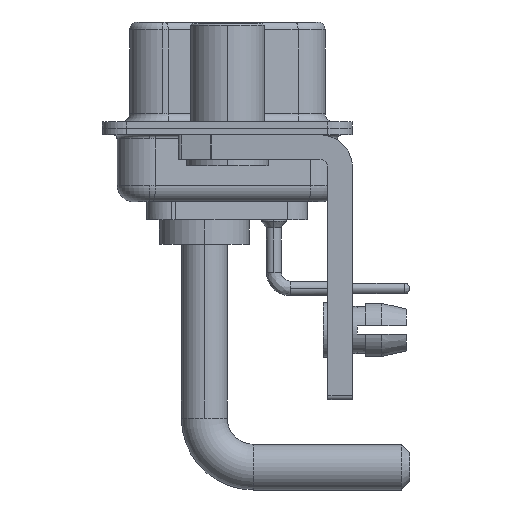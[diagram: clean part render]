
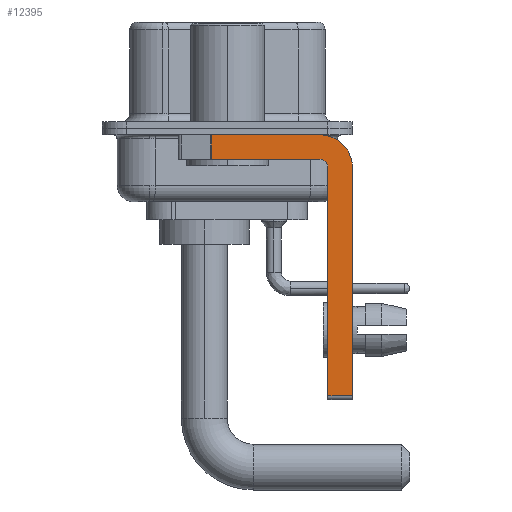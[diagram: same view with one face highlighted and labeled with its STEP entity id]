
A CAD part, left-side view. The second image highlights one B-rep face of the part: STEP entity #12395.
In plain terms, the highlighted planar face has unit normal (-1, 0, 0).
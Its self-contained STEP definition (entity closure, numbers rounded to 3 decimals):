
#335 = VECTOR ( 'NONE', #17291, 1000. ) ;
#448 = VECTOR ( 'NONE', #26796, 1000. ) ;
#1415 = AXIS2_PLACEMENT_3D ( 'NONE', #9106, #7121, #15744 ) ;
#1646 = LINE ( 'NONE', #10288, #11761 ) ;
#1775 = CARTESIAN_POINT ( 'NONE',  ( -2.9, -7.65, -2.4 ) ) ;
#2487 = ORIENTED_EDGE ( 'NONE', *, *, #11642, .F. ) ;
#3625 = AXIS2_PLACEMENT_3D ( 'NONE', #11857, #13549, #9172 ) ;
#4670 = LINE ( 'NONE', #25917, #10316 ) ;
#4690 = VERTEX_POINT ( 'NONE', #8998 ) ;
#4702 = EDGE_CURVE ( 'NONE', #9574, #25450, #22022, .T. ) ;
#4993 = CIRCLE ( 'NONE', #1415, 2. ) ;
#5126 = VERTEX_POINT ( 'NONE', #18393 ) ;
#7117 = EDGE_LOOP ( 'NONE', ( #9124, #17147, #12365, #19292, #2487, #23918, #9658, #9670 ) ) ;
#7121 = DIRECTION ( 'NONE',  ( 1., 0., 0. ) ) ;
#7464 = PLANE ( 'NONE',  #3625 ) ;
#8009 = DIRECTION ( 'NONE',  ( -1., 0., 0. ) ) ;
#8576 = DIRECTION ( 'NONE',  ( 0., -1., 0. ) ) ;
#8673 = CARTESIAN_POINT ( 'NONE',  ( -2.9, -5.65, -16.35 ) ) ;
#8998 = CARTESIAN_POINT ( 'NONE',  ( -2.9, 0.978, -1.9 ) ) ;
#9106 = CARTESIAN_POINT ( 'NONE',  ( -2.9, -5.65, -2.4 ) ) ;
#9124 = ORIENTED_EDGE ( 'NONE', *, *, #13125, .F. ) ;
#9172 = DIRECTION ( 'NONE',  ( 0., 0., -1. ) ) ;
#9574 = VERTEX_POINT ( 'NONE', #1775 ) ;
#9658 = ORIENTED_EDGE ( 'NONE', *, *, #4702, .F. ) ;
#9670 = ORIENTED_EDGE ( 'NONE', *, *, #26041, .F. ) ;
#10172 = VERTEX_POINT ( 'NONE', #19708 ) ;
#10288 = CARTESIAN_POINT ( 'NONE',  ( -2.9, 3., -0.4 ) ) ;
#10316 = VECTOR ( 'NONE', #13300, 1000. ) ;
#11395 = VERTEX_POINT ( 'NONE', #25543 ) ;
#11642 = EDGE_CURVE ( 'NONE', #5126, #10172, #13886, .T. ) ;
#11761 = VECTOR ( 'NONE', #8576, 1000. ) ;
#11857 = CARTESIAN_POINT ( 'NONE',  ( -2.9, -5.65, -2.4 ) ) ;
#11961 = DIRECTION ( 'NONE',  ( 0., 0., -1. ) ) ;
#12365 = ORIENTED_EDGE ( 'NONE', *, *, #17684, .F. ) ;
#12395 = ADVANCED_FACE ( 'NONE', ( #20202 ), #7464, .F. ) ;
#13125 = EDGE_CURVE ( 'NONE', #26053, #11395, #1646, .T. ) ;
#13178 = VECTOR ( 'NONE', #11961, 1000. ) ;
#13300 = DIRECTION ( 'NONE',  ( 0., 1., 0. ) ) ;
#13549 = DIRECTION ( 'NONE',  ( 1., 0., 0. ) ) ;
#13759 = CARTESIAN_POINT ( 'NONE',  ( -2.9, -6.15, -16.6 ) ) ;
#13886 = LINE ( 'NONE', #13759, #448 ) ;
#15744 = DIRECTION ( 'NONE',  ( 0., 0., -1. ) ) ;
#15843 = EDGE_CURVE ( 'NONE', #26053, #4690, #19353, .T. ) ;
#15903 = VECTOR ( 'NONE', #26146, 1000. ) ;
#17147 = ORIENTED_EDGE ( 'NONE', *, *, #15843, .T. ) ;
#17173 = EDGE_CURVE ( 'NONE', #5126, #25450, #26367, .T. ) ;
#17198 = CARTESIAN_POINT ( 'NONE',  ( -2.9, -7.65, -16.35 ) ) ;
#17291 = DIRECTION ( 'NONE',  ( 0., -1., 0. ) ) ;
#17684 = EDGE_CURVE ( 'NONE', #19979, #4690, #4670, .T. ) ;
#18155 = CARTESIAN_POINT ( 'NONE',  ( -2.9, 0.978, -0.4 ) ) ;
#18393 = CARTESIAN_POINT ( 'NONE',  ( -2.9, -6.15, -16.35 ) ) ;
#18909 = CARTESIAN_POINT ( 'NONE',  ( -2.9, -5.65, -2.4 ) ) ;
#19292 = ORIENTED_EDGE ( 'NONE', *, *, #23927, .F. ) ;
#19353 = LINE ( 'NONE', #24034, #15903 ) ;
#19708 = CARTESIAN_POINT ( 'NONE',  ( -2.9, -6.15, -2.4 ) ) ;
#19979 = VERTEX_POINT ( 'NONE', #25011 ) ;
#20202 = FACE_OUTER_BOUND ( 'NONE', #7117, .T. ) ;
#22022 = LINE ( 'NONE', #25128, #13178 ) ;
#22883 = DIRECTION ( 'NONE',  ( 0., 0., 1. ) ) ;
#23918 = ORIENTED_EDGE ( 'NONE', *, *, #17173, .T. ) ;
#23927 = EDGE_CURVE ( 'NONE', #10172, #19979, #24711, .T. ) ;
#24034 = CARTESIAN_POINT ( 'NONE',  ( -2.9, 0.978, -1.9 ) ) ;
#24711 = CIRCLE ( 'NONE', #27431, 0.5 ) ;
#25011 = CARTESIAN_POINT ( 'NONE',  ( -2.9, -5.65, -1.9 ) ) ;
#25128 = CARTESIAN_POINT ( 'NONE',  ( -2.9, -7.65, -2.4 ) ) ;
#25450 = VERTEX_POINT ( 'NONE', #17198 ) ;
#25543 = CARTESIAN_POINT ( 'NONE',  ( -2.9, -5.65, -0.4 ) ) ;
#25917 = CARTESIAN_POINT ( 'NONE',  ( -2.9, -5.65, -1.9 ) ) ;
#26041 = EDGE_CURVE ( 'NONE', #11395, #9574, #4993, .T. ) ;
#26053 = VERTEX_POINT ( 'NONE', #18155 ) ;
#26146 = DIRECTION ( 'NONE',  ( 0., 0., -1. ) ) ;
#26367 = LINE ( 'NONE', #8673, #335 ) ;
#26796 = DIRECTION ( 'NONE',  ( 0., 0., 1. ) ) ;
#27431 = AXIS2_PLACEMENT_3D ( 'NONE', #18909, #8009, #22883 ) ;
